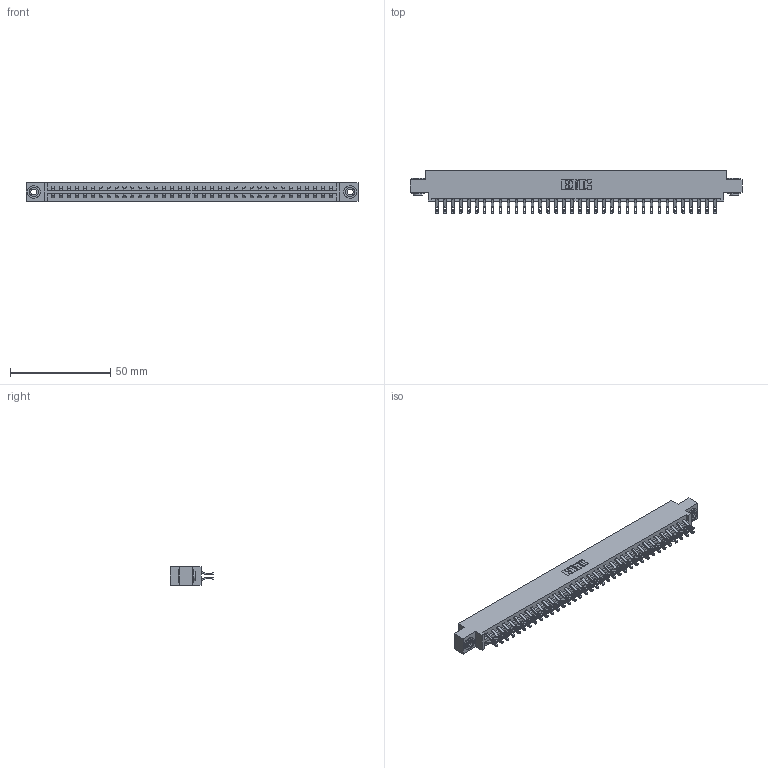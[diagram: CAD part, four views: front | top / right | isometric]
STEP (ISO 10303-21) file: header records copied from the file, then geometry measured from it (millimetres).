
FILE_DESCRIPTION (( 'STEP AP203' ), '1' );
FILE_NAME ('337-072-555-803.STEP', '2019-10-15T11:52:12', ( '' ), ( '' ), 'SwSTEP 2.0', 'SolidWorks 2016', '' );
FILE_SCHEMA (( 'CONFIG_CONTROL_DESIGN' ));
Length unit declared in the file: inch
Products named in the file (4): 337-072-555-803; 345-250-002_345-250-002-102; 345-292-001_555 Tail; 337 Part_0.170 Offset - 0.156 Dia-TH
Assembly tree (75 placements, depth 2):
  337-072-555-803
    337 Part_0.170 Offset - 0.156 Dia-TH
    345-292-001_555 Tail  x72
    345-250-002_345-250-002-102  x2
Bounding box: 165.66 x 21.47 x 9.4 mm (x, y, z)
Volume: 17489.3 mm3; surface area: 20832.7 mm2
Topology: 75 solids, 75 shells, 4476 faces, 14007 edges, 9334 vertices
Faces by surface type: plane 2676, cylinder 1792, cone 8
Entity records: 29796 total; most frequent: CARTESIAN_POINT 5035, ORIENTED_EDGE 4934, DIRECTION 4297, EDGE_CURVE 2467, VECTOR 2295, LINE 2295, VERTEX_POINT 1642, AXIS2_PLACEMENT_3D 1001
